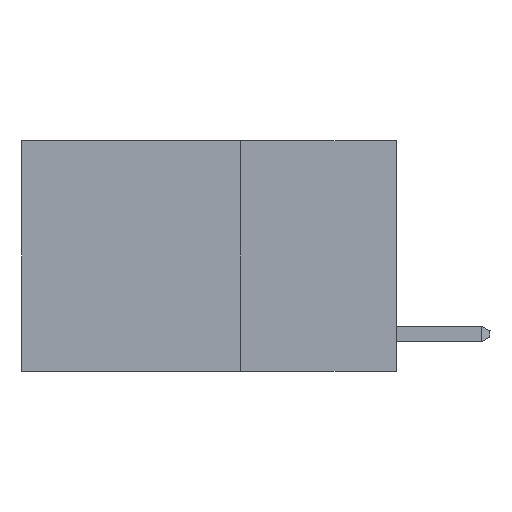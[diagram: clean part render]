
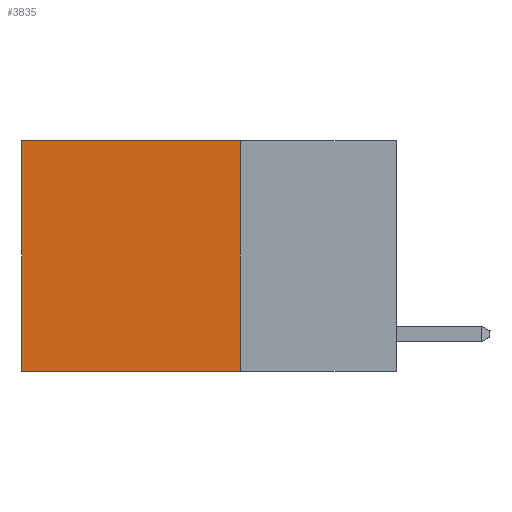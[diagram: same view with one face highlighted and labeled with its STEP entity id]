
A CAD part, left-side view. The second image highlights one B-rep face of the part: STEP entity #3835.
In plain terms, the highlighted planar face has unit normal (-1, 0, 0).
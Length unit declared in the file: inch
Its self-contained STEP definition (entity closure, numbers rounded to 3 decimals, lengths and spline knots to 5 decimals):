
#1259 = CARTESIAN_POINT ( 'NONE',  ( 0.2625, 0.25, -0.37 ) ) ;
#2243 = DIRECTION ( 'NONE',  ( 0., 0., -1. ) ) ;
#2874 = DIRECTION ( 'NONE',  ( 0., 0., -1. ) ) ;
#2906 = LINE ( 'NONE', #5666, #11456 ) ;
#2949 = AXIS2_PLACEMENT_3D ( 'NONE', #13680, #13799, #2874 ) ;
#3020 = FACE_OUTER_BOUND ( 'NONE', #14790, .T. ) ;
#3669 = EDGE_CURVE ( 'NONE', #5825, #16787, #4353, .T. ) ;
#3835 = ADVANCED_FACE ( 'NONE', ( #3020 ), #3938, .F. ) ;
#3938 = PLANE ( 'NONE',  #2949 ) ;
#4281 = CARTESIAN_POINT ( 'NONE',  ( 0.2625, 0.25, 0. ) ) ;
#4353 = LINE ( 'NONE', #15026, #14486 ) ;
#4494 = VECTOR ( 'NONE', #6778, 39.37008 ) ;
#5666 = CARTESIAN_POINT ( 'NONE',  ( 0.2625, 0.25, -0.37 ) ) ;
#5825 = VERTEX_POINT ( 'NONE', #13315 ) ;
#6778 = DIRECTION ( 'NONE',  ( 0., 1., 0. ) ) ;
#7954 = VERTEX_POINT ( 'NONE', #1259 ) ;
#8149 = EDGE_CURVE ( 'NONE', #7954, #16787, #2906, .T. ) ;
#8553 = DIRECTION ( 'NONE',  ( 0., 0., -1. ) ) ;
#10102 = CARTESIAN_POINT ( 'NONE',  ( 0.2625, 0.25, 0. ) ) ;
#11265 = ORIENTED_EDGE ( 'NONE', *, *, #15543, .F. ) ;
#11456 = VECTOR ( 'NONE', #15558, 39.37008 ) ;
#11834 = ORIENTED_EDGE ( 'NONE', *, *, #3669, .T. ) ;
#12160 = VERTEX_POINT ( 'NONE', #10102 ) ;
#12184 = VECTOR ( 'NONE', #8553, 39.37008 ) ;
#12400 = CARTESIAN_POINT ( 'NONE',  ( 0.2625, 0.25, 0. ) ) ;
#13315 = CARTESIAN_POINT ( 'NONE',  ( 0.2625, 0.6, 0. ) ) ;
#13680 = CARTESIAN_POINT ( 'NONE',  ( 0.2625, 0.25, 0. ) ) ;
#13799 = DIRECTION ( 'NONE',  ( 1., 0., 0. ) ) ;
#13970 = LINE ( 'NONE', #12400, #4494 ) ;
#14078 = CARTESIAN_POINT ( 'NONE',  ( 0.2625, 0.6, -0.37 ) ) ;
#14486 = VECTOR ( 'NONE', #2243, 39.37008 ) ;
#14790 = EDGE_LOOP ( 'NONE', ( #11834, #16379, #11265, #18257 ) ) ;
#15026 = CARTESIAN_POINT ( 'NONE',  ( 0.2625, 0.6, 0. ) ) ;
#15543 = EDGE_CURVE ( 'NONE', #12160, #7954, #15949, .T. ) ;
#15558 = DIRECTION ( 'NONE',  ( 0., 1., 0. ) ) ;
#15931 = EDGE_CURVE ( 'NONE', #12160, #5825, #13970, .T. ) ;
#15949 = LINE ( 'NONE', #4281, #12184 ) ;
#16379 = ORIENTED_EDGE ( 'NONE', *, *, #8149, .F. ) ;
#16787 = VERTEX_POINT ( 'NONE', #14078 ) ;
#18257 = ORIENTED_EDGE ( 'NONE', *, *, #15931, .T. ) ;
